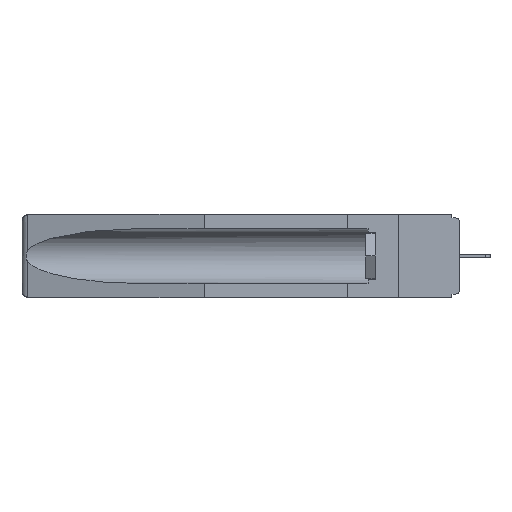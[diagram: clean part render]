
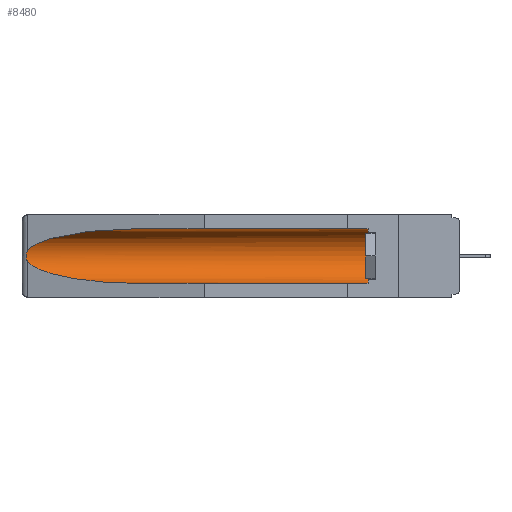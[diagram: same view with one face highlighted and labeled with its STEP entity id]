
A CAD part, left-side view. The second image highlights one B-rep face of the part: STEP entity #8480.
In plain terms, the highlighted cylindrical face has radius 2.857 mm (diameter 5.715 mm), a partial arc.
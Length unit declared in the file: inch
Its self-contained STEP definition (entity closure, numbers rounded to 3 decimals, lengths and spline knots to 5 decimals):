
#33 = ORIENTED_EDGE ( 'NONE', *, *, #3960, .T. ) ;
#42 = VERTEX_POINT ( 'NONE', #3436 ) ;
#151 = LINE ( 'NONE', #15655, #13577 ) ;
#196 = DIRECTION ( 'NONE',  ( 0., 1., 0. ) ) ;
#441 = ORIENTED_EDGE ( 'NONE', *, *, #6523, .T. ) ;
#494 = CARTESIAN_POINT ( 'NONE',  ( 0.2675, 1.53308, -0.16763 ) ) ;
#973 = DIRECTION ( 'NONE',  ( 0., 0., 1. ) ) ;
#976 = CARTESIAN_POINT ( 'NONE',  ( 0.25451, 1.48313, -0.24835 ) ) ;
#1591 =( BOUNDED_CURVE ( )  B_SPLINE_CURVE ( 3, ( #11336, #976, #2361, #12658 ),
 .UNSPECIFIED., .F., .F. ) 
 B_SPLINE_CURVE_WITH_KNOTS ( ( 4, 4 ),
 ( 0.1948, 1.5708 ),
 .UNSPECIFIED. ) 
 CURVE ( )  GEOMETRIC_REPRESENTATION_ITEM ( )  RATIONAL_B_SPLINE_CURVE ( ( 1., 0.848, 0.848, 1. ) ) 
 REPRESENTATION_ITEM ( '' )  );
#1892 = CARTESIAN_POINT ( 'NONE',  ( 0.2673, 1.53269, -0.17917 ) ) ;
#2361 = CARTESIAN_POINT ( 'NONE',  ( 0.21114, 1.30732, -0.284 ) ) ;
#2366 = CYLINDRICAL_SURFACE ( 'NONE', #4090, 0.1125 ) ;
#2715 = AXIS2_PLACEMENT_3D ( 'NONE', #6737, #15607, #7999 ) ;
#3229 = CARTESIAN_POINT ( 'NONE',  ( 0.26597, 1.5296, -0.19026 ) ) ;
#3238 = ORIENTED_EDGE ( 'NONE', *, *, #15408, .F. ) ;
#3436 = CARTESIAN_POINT ( 'NONE',  ( 0.26537, 1.52718, -0.14972 ) ) ;
#3960 = EDGE_CURVE ( 'NONE', #11428, #8817, #10938, .T. ) ;
#3995 = EDGE_CURVE ( 'NONE', #8817, #12952, #151, .T. ) ;
#4090 = AXIS2_PLACEMENT_3D ( 'NONE', #7499, #10016, #973 ) ;
#5386 = CARTESIAN_POINT ( 'NONE',  ( 0.155, -0.30754, -0.284 ) ) ;
#5639 = EDGE_LOOP ( 'NONE', ( #441, #8573, #7994, #3238, #33, #14295 ) ) ;
#6061 = CARTESIAN_POINT ( 'NONE',  ( 0.21114, 1.30732, -0.059 ) ) ;
#6227 = FACE_OUTER_BOUND ( 'NONE', #5639, .T. ) ;
#6523 = EDGE_CURVE ( 'NONE', #12952, #42, #15250, .T. ) ;
#6609 = EDGE_CURVE ( 'NONE', #14782, #10834, #1591, .T. ) ;
#6737 = CARTESIAN_POINT ( 'NONE',  ( 0.155, 0.126, -0.1715 ) ) ;
#7493 = CARTESIAN_POINT ( 'NONE',  ( 0.155, 1.07973, -0.284 ) ) ;
#7499 = CARTESIAN_POINT ( 'NONE',  ( 0.155, -0.30754, -0.1715 ) ) ;
#7865 = DIRECTION ( 'NONE',  ( 0., 1., 0. ) ) ;
#7994 = ORIENTED_EDGE ( 'NONE', *, *, #6609, .T. ) ;
#7999 = DIRECTION ( 'NONE',  ( 0., 0., 1. ) ) ;
#8275 = CARTESIAN_POINT ( 'NONE',  ( 0.26597, 1.52961, -0.15275 ) ) ;
#8330 = CARTESIAN_POINT ( 'NONE',  ( 0.2673, 1.5327, -0.16383 ) ) ;
#8480 = ADVANCED_FACE ( 'NONE', ( #6227 ), #2366, .F. ) ;
#8573 = ORIENTED_EDGE ( 'NONE', *, *, #13757, .T. ) ;
#8587 = CARTESIAN_POINT ( 'NONE',  ( 0.26537, 1.52718, -0.14972 ) ) ;
#8817 = VERTEX_POINT ( 'NONE', #14744 ) ;
#9575 = CARTESIAN_POINT ( 'NONE',  ( 0.2675, 1.53308, -0.17534 ) ) ;
#9868 = CARTESIAN_POINT ( 'NONE',  ( 0.155, 0.126, -0.284 ) ) ;
#10010 = B_SPLINE_CURVE_WITH_KNOTS ( 'NONE', 3,
 ( #14706, #8275, #15921, #8330, #494, #9575, #1892, #10879, #3229, #12195 ),
 .UNSPECIFIED., .F., .F.,
 ( 4, 2, 2, 2, 4 ),
 ( 0., 0.00029, 0.00058, 0.00087, 0.00117 ),
 .UNSPECIFIED. ) ;
#10016 = DIRECTION ( 'NONE',  ( 0., 1., 0. ) ) ;
#10742 = LINE ( 'NONE', #5386, #14182 ) ;
#10834 = VERTEX_POINT ( 'NONE', #7493 ) ;
#10879 = CARTESIAN_POINT ( 'NONE',  ( 0.26655, 1.53094, -0.18657 ) ) ;
#10938 = CIRCLE ( 'NONE', #2715, 0.1125 ) ;
#11336 = CARTESIAN_POINT ( 'NONE',  ( 0.26537, 1.52718, -0.19328 ) ) ;
#11428 = VERTEX_POINT ( 'NONE', #9868 ) ;
#12195 = CARTESIAN_POINT ( 'NONE',  ( 0.26537, 1.52718, -0.19328 ) ) ;
#12421 = CARTESIAN_POINT ( 'NONE',  ( 0.155, 1.07973, -0.059 ) ) ;
#12658 = CARTESIAN_POINT ( 'NONE',  ( 0.155, 1.07973, -0.284 ) ) ;
#12836 = CARTESIAN_POINT ( 'NONE',  ( 0.26537, 1.52718, -0.19328 ) ) ;
#12952 = VERTEX_POINT ( 'NONE', #14355 ) ;
#13577 = VECTOR ( 'NONE', #196, 39.37008 ) ;
#13757 = EDGE_CURVE ( 'NONE', #42, #14782, #10010, .T. ) ;
#14182 = VECTOR ( 'NONE', #7865, 39.37008 ) ;
#14295 = ORIENTED_EDGE ( 'NONE', *, *, #3995, .T. ) ;
#14355 = CARTESIAN_POINT ( 'NONE',  ( 0.155, 1.07973, -0.059 ) ) ;
#14706 = CARTESIAN_POINT ( 'NONE',  ( 0.26537, 1.52718, -0.14972 ) ) ;
#14744 = CARTESIAN_POINT ( 'NONE',  ( 0.155, 0.126, -0.059 ) ) ;
#14782 = VERTEX_POINT ( 'NONE', #12836 ) ;
#15250 =( BOUNDED_CURVE ( )  B_SPLINE_CURVE ( 3, ( #12421, #6061, #16171, #8587 ),
 .UNSPECIFIED., .F., .F. ) 
 B_SPLINE_CURVE_WITH_KNOTS ( ( 4, 4 ),
 ( 4.71239, 6.08839 ),
 .UNSPECIFIED. ) 
 CURVE ( )  GEOMETRIC_REPRESENTATION_ITEM ( )  RATIONAL_B_SPLINE_CURVE ( ( 1., 0.848, 0.848, 1. ) ) 
 REPRESENTATION_ITEM ( '' )  );
#15408 = EDGE_CURVE ( 'NONE', #11428, #10834, #10742, .T. ) ;
#15607 = DIRECTION ( 'NONE',  ( 0., -1., 0. ) ) ;
#15655 = CARTESIAN_POINT ( 'NONE',  ( 0.155, -0.30754, -0.059 ) ) ;
#15921 = CARTESIAN_POINT ( 'NONE',  ( 0.26654, 1.53092, -0.15636 ) ) ;
#16171 = CARTESIAN_POINT ( 'NONE',  ( 0.25451, 1.48313, -0.09465 ) ) ;
